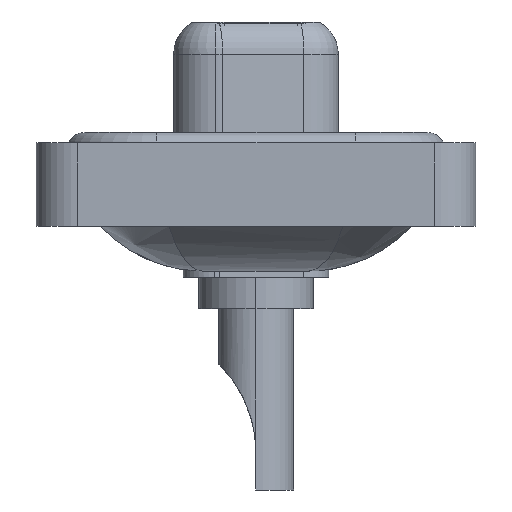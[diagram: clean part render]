
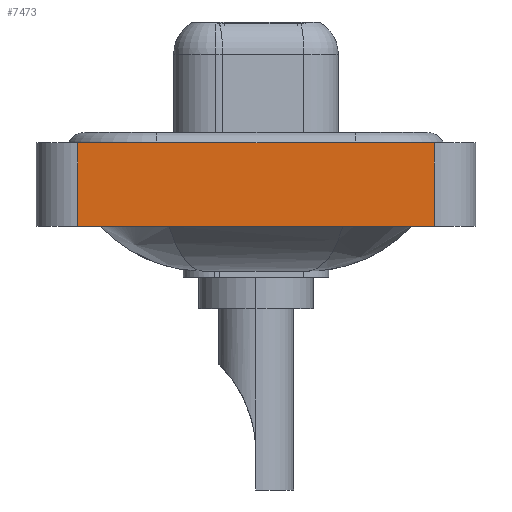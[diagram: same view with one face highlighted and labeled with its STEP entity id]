
A CAD part, left-side view. The second image highlights one B-rep face of the part: STEP entity #7473.
In plain terms, the highlighted planar face has unit normal (-1, 0, 0).
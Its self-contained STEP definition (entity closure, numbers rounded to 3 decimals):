
#136 = VECTOR ( 'NONE', #344, 1000. ) ;
#344 = DIRECTION ( 'NONE',  ( 0., -1., 0. ) ) ;
#1493 = CARTESIAN_POINT ( 'NONE',  ( -7.3, -8.55, -3.6 ) ) ;
#2005 = PLANE ( 'NONE',  #13228 ) ;
#2874 = CARTESIAN_POINT ( 'NONE',  ( -7.3, -8.55, -3.6 ) ) ;
#2960 = DIRECTION ( 'NONE',  ( 0., -1., 0. ) ) ;
#3337 = DIRECTION ( 'NONE',  ( -1., 0., 0. ) ) ;
#3486 = VERTEX_POINT ( 'NONE', #1493 ) ;
#4399 = VERTEX_POINT ( 'NONE', #6323 ) ;
#4596 = DIRECTION ( 'NONE',  ( 0., 0., 1. ) ) ;
#5128 = VECTOR ( 'NONE', #15846, 1000. ) ;
#5253 = VERTEX_POINT ( 'NONE', #5823 ) ;
#5296 = EDGE_LOOP ( 'NONE', ( #16070, #14722, #15230, #10261 ) ) ;
#5717 = LINE ( 'NONE', #2874, #14694 ) ;
#5823 = CARTESIAN_POINT ( 'NONE',  ( -7.3, 8.55, -3.6 ) ) ;
#5973 = VERTEX_POINT ( 'NONE', #8903 ) ;
#6323 = CARTESIAN_POINT ( 'NONE',  ( -7.3, -8.55, 0.4 ) ) ;
#7088 = CARTESIAN_POINT ( 'NONE',  ( -7.3, -8.55, -3.6 ) ) ;
#7207 = VECTOR ( 'NONE', #4596, 1000. ) ;
#7473 = ADVANCED_FACE ( 'NONE', ( #13396 ), #2005, .T. ) ;
#7823 = LINE ( 'NONE', #10306, #136 ) ;
#8266 = LINE ( 'NONE', #13319, #7207 ) ;
#8392 = LINE ( 'NONE', #11964, #5128 ) ;
#8666 = EDGE_CURVE ( 'NONE', #5253, #3486, #5717, .T. ) ;
#8903 = CARTESIAN_POINT ( 'NONE',  ( -7.3, 8.55, 0.4 ) ) ;
#9517 = EDGE_CURVE ( 'NONE', #5973, #4399, #7823, .T. ) ;
#10261 = ORIENTED_EDGE ( 'NONE', *, *, #8666, .T. ) ;
#10306 = CARTESIAN_POINT ( 'NONE',  ( -7.3, -8.55, 0.4 ) ) ;
#11909 = DIRECTION ( 'NONE',  ( 0., 0., 1. ) ) ;
#11931 = EDGE_CURVE ( 'NONE', #3486, #4399, #8266, .T. ) ;
#11964 = CARTESIAN_POINT ( 'NONE',  ( -7.3, 8.55, -3.6 ) ) ;
#12984 = EDGE_CURVE ( 'NONE', #5253, #5973, #8392, .T. ) ;
#13228 = AXIS2_PLACEMENT_3D ( 'NONE', #7088, #3337, #11909 ) ;
#13319 = CARTESIAN_POINT ( 'NONE',  ( -7.3, -8.55, -3.6 ) ) ;
#13396 = FACE_OUTER_BOUND ( 'NONE', #5296, .T. ) ;
#14694 = VECTOR ( 'NONE', #2960, 1000. ) ;
#14722 = ORIENTED_EDGE ( 'NONE', *, *, #9517, .F. ) ;
#15230 = ORIENTED_EDGE ( 'NONE', *, *, #12984, .F. ) ;
#15846 = DIRECTION ( 'NONE',  ( 0., 0., 1. ) ) ;
#16070 = ORIENTED_EDGE ( 'NONE', *, *, #11931, .T. ) ;
